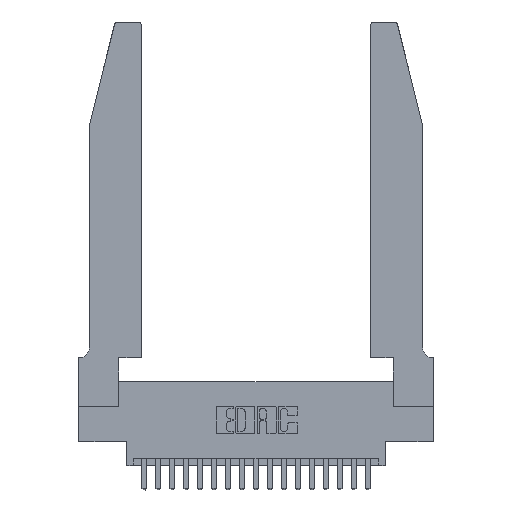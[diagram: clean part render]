
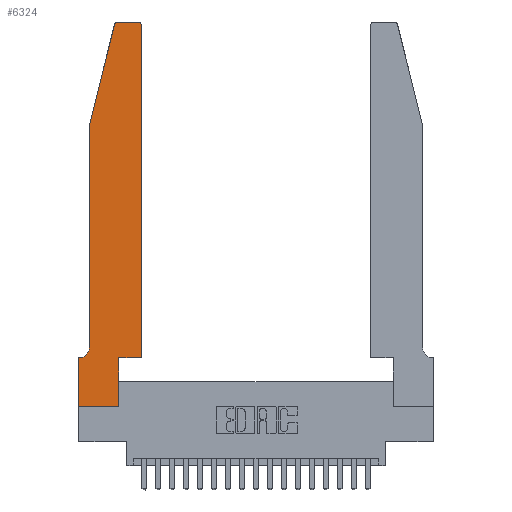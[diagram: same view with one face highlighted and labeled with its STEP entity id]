
A CAD part, top view. The second image highlights one B-rep face of the part: STEP entity #6324.
In plain terms, the highlighted planar face has unit normal (0, 0, 1).
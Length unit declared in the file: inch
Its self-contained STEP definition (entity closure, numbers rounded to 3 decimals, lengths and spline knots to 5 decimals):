
#90 = DIRECTION ( 'NONE',  ( -1., 0., 0. ) ) ;
#198 = LINE ( 'NONE', #14438, #8178 ) ;
#843 = ORIENTED_EDGE ( 'NONE', *, *, #17183, .T. ) ;
#995 = EDGE_CURVE ( 'NONE', #16511, #7990, #11975, .T. ) ;
#1107 = EDGE_CURVE ( 'NONE', #16367, #17988, #9877, .T. ) ;
#1293 = VECTOR ( 'NONE', #10510, 39.37008 ) ;
#1781 = DIRECTION ( 'NONE',  ( 0., 1., 0. ) ) ;
#1862 = EDGE_CURVE ( 'NONE', #20897, #2312, #12445, .T. ) ;
#1944 = CARTESIAN_POINT ( 'NONE',  ( 0.2865, 0.35, 0.37 ) ) ;
#2169 = DIRECTION ( 'NONE',  ( 0., 0., 1. ) ) ;
#2183 = CARTESIAN_POINT ( 'NONE',  ( 0.2865, 0., 0.37 ) ) ;
#2267 = AXIS2_PLACEMENT_3D ( 'NONE', #20185, #10224, #90 ) ;
#2312 = VERTEX_POINT ( 'NONE', #20329 ) ;
#2455 = ORIENTED_EDGE ( 'NONE', *, *, #7829, .T. ) ;
#3003 = VECTOR ( 'NONE', #5494, 39.37008 ) ;
#3205 = CARTESIAN_POINT ( 'NONE',  ( 0.2605, 2.75, 0.37 ) ) ;
#3288 = DIRECTION ( 'NONE',  ( -1., 0., 0. ) ) ;
#3843 = DIRECTION ( 'NONE',  ( 1., 0., 0. ) ) ;
#3887 = LINE ( 'NONE', #7408, #21116 ) ;
#4576 = EDGE_LOOP ( 'NONE', ( #19157, #11309, #12331, #10858, #843, #12430, #13785, #2455, #6775, #19074, #5252, #10156 ) ) ;
#4817 = CARTESIAN_POINT ( 'NONE',  ( 0.4505, 2.72, 0.37 ) ) ;
#5075 = LINE ( 'NONE', #3205, #8491 ) ;
#5190 = EDGE_CURVE ( 'NONE', #17258, #20897, #198, .T. ) ;
#5252 = ORIENTED_EDGE ( 'NONE', *, *, #5190, .T. ) ;
#5332 = LINE ( 'NONE', #20556, #1293 ) ;
#5494 = DIRECTION ( 'NONE',  ( 0., -1., 0. ) ) ;
#5648 = CARTESIAN_POINT ( 'NONE',  ( 0.0755, 2., 0.37 ) ) ;
#5814 = DIRECTION ( 'NONE',  ( 0., 0., 1. ) ) ;
#6324 = ADVANCED_FACE ( 'NONE', ( #13847 ), #20495, .T. ) ;
#6396 = EDGE_CURVE ( 'NONE', #11223, #14682, #3887, .T. ) ;
#6482 = VERTEX_POINT ( 'NONE', #20991 ) ;
#6564 = EDGE_CURVE ( 'NONE', #7552, #15938, #9677, .T. ) ;
#6672 = DIRECTION ( 'NONE',  ( -0.239, -0.971, 0. ) ) ;
#6775 = ORIENTED_EDGE ( 'NONE', *, *, #1107, .T. ) ;
#7034 = CARTESIAN_POINT ( 'NONE',  ( 0., 0.35, 0.37 ) ) ;
#7202 = CIRCLE ( 'NONE', #2267, 0.07 ) ;
#7408 = CARTESIAN_POINT ( 'NONE',  ( 0.0755, 0.35, 0.37 ) ) ;
#7552 = VERTEX_POINT ( 'NONE', #13326 ) ;
#7829 = EDGE_CURVE ( 'NONE', #6482, #16367, #5332, .T. ) ;
#7989 = CARTESIAN_POINT ( 'NONE',  ( 0.284, 2.72, 0.37 ) ) ;
#7990 = VERTEX_POINT ( 'NONE', #10951 ) ;
#8178 = VECTOR ( 'NONE', #16109, 39.37008 ) ;
#8262 = CARTESIAN_POINT ( 'NONE',  ( 0.0755, 2., 0.37 ) ) ;
#8491 = VECTOR ( 'NONE', #3288, 39.37008 ) ;
#9498 = CARTESIAN_POINT ( 'NONE',  ( 0.0055, 0.35, 0.37 ) ) ;
#9656 = DIRECTION ( 'NONE',  ( 1., 0., 0. ) ) ;
#9677 = CIRCLE ( 'NONE', #21260, 0.03 ) ;
#9877 = LINE ( 'NONE', #1944, #10380 ) ;
#10138 = LINE ( 'NONE', #8262, #14036 ) ;
#10156 = ORIENTED_EDGE ( 'NONE', *, *, #1862, .T. ) ;
#10224 = DIRECTION ( 'NONE',  ( 0., 0., -1. ) ) ;
#10380 = VECTOR ( 'NONE', #1781, 39.37008 ) ;
#10510 = DIRECTION ( 'NONE',  ( 1., 0., 0. ) ) ;
#10539 = CARTESIAN_POINT ( 'NONE',  ( 0.2865, 0.35, 0.37 ) ) ;
#10858 = ORIENTED_EDGE ( 'NONE', *, *, #995, .T. ) ;
#10951 = CARTESIAN_POINT ( 'NONE',  ( 0.0755, 0.42, 0.37 ) ) ;
#11223 = VERTEX_POINT ( 'NONE', #9498 ) ;
#11309 = ORIENTED_EDGE ( 'NONE', *, *, #6564, .T. ) ;
#11546 = CARTESIAN_POINT ( 'NONE',  ( 0.4505, 0.35, 0.37 ) ) ;
#11975 = LINE ( 'NONE', #5648, #3003 ) ;
#12290 = CARTESIAN_POINT ( 'NONE',  ( 0., 0.35, 0.37 ) ) ;
#12331 = ORIENTED_EDGE ( 'NONE', *, *, #15348, .T. ) ;
#12430 = ORIENTED_EDGE ( 'NONE', *, *, #6396, .T. ) ;
#12445 = CIRCLE ( 'NONE', #21487, 0.03 ) ;
#12809 = CARTESIAN_POINT ( 'NONE',  ( 0.0755, 2., 0.37 ) ) ;
#13222 = DIRECTION ( 'NONE',  ( 1., 0., 0. ) ) ;
#13326 = CARTESIAN_POINT ( 'NONE',  ( 0.284, 2.75, 0.37 ) ) ;
#13652 = CARTESIAN_POINT ( 'NONE',  ( 0.4505, 0.35, 0.37 ) ) ;
#13739 = CARTESIAN_POINT ( 'NONE',  ( 0.4205, 2.72, 0.37 ) ) ;
#13785 = ORIENTED_EDGE ( 'NONE', *, *, #17689, .T. ) ;
#13847 = FACE_OUTER_BOUND ( 'NONE', #4576, .T. ) ;
#13954 = DIRECTION ( 'NONE',  ( 1., 0., 0. ) ) ;
#14036 = VECTOR ( 'NONE', #6672, 39.37008 ) ;
#14438 = CARTESIAN_POINT ( 'NONE',  ( 0.4505, 0.35, 0.37 ) ) ;
#14682 = VERTEX_POINT ( 'NONE', #7034 ) ;
#15000 = VECTOR ( 'NONE', #18003, 39.37008 ) ;
#15101 = VECTOR ( 'NONE', #13222, 39.37008 ) ;
#15309 = EDGE_CURVE ( 'NONE', #17988, #17258, #15603, .T. ) ;
#15348 = EDGE_CURVE ( 'NONE', #15938, #16511, #10138, .T. ) ;
#15603 = LINE ( 'NONE', #11546, #15101 ) ;
#15761 = DIRECTION ( 'NONE',  ( -1., 0., 0. ) ) ;
#15938 = VERTEX_POINT ( 'NONE', #16400 ) ;
#16031 = LINE ( 'NONE', #16323, #15000 ) ;
#16109 = DIRECTION ( 'NONE',  ( 0., 1., 0. ) ) ;
#16323 = CARTESIAN_POINT ( 'NONE',  ( 0., 0., 0.37 ) ) ;
#16367 = VERTEX_POINT ( 'NONE', #2183 ) ;
#16400 = CARTESIAN_POINT ( 'NONE',  ( 0.25487, 2.72718, 0.37 ) ) ;
#16511 = VERTEX_POINT ( 'NONE', #12809 ) ;
#17183 = EDGE_CURVE ( 'NONE', #7990, #11223, #7202, .T. ) ;
#17258 = VERTEX_POINT ( 'NONE', #13652 ) ;
#17689 = EDGE_CURVE ( 'NONE', #14682, #6482, #16031, .T. ) ;
#17807 = EDGE_CURVE ( 'NONE', #2312, #7552, #5075, .T. ) ;
#17988 = VERTEX_POINT ( 'NONE', #10539 ) ;
#18003 = DIRECTION ( 'NONE',  ( 0., -1., 0. ) ) ;
#19074 = ORIENTED_EDGE ( 'NONE', *, *, #15309, .T. ) ;
#19157 = ORIENTED_EDGE ( 'NONE', *, *, #17807, .T. ) ;
#19616 = DIRECTION ( 'NONE',  ( 0., 0., 1. ) ) ;
#20185 = CARTESIAN_POINT ( 'NONE',  ( 0.0055, 0.42, 0.37 ) ) ;
#20329 = CARTESIAN_POINT ( 'NONE',  ( 0.4205, 2.75, 0.37 ) ) ;
#20495 = PLANE ( 'NONE',  #21688 ) ;
#20556 = CARTESIAN_POINT ( 'NONE',  ( 0., 0., 0.37 ) ) ;
#20897 = VERTEX_POINT ( 'NONE', #4817 ) ;
#20991 = CARTESIAN_POINT ( 'NONE',  ( 0., 0., 0.37 ) ) ;
#21116 = VECTOR ( 'NONE', #15761, 39.37008 ) ;
#21260 = AXIS2_PLACEMENT_3D ( 'NONE', #7989, #19616, #9656 ) ;
#21487 = AXIS2_PLACEMENT_3D ( 'NONE', #13739, #5814, #3843 ) ;
#21688 = AXIS2_PLACEMENT_3D ( 'NONE', #12290, #2169, #13954 ) ;
